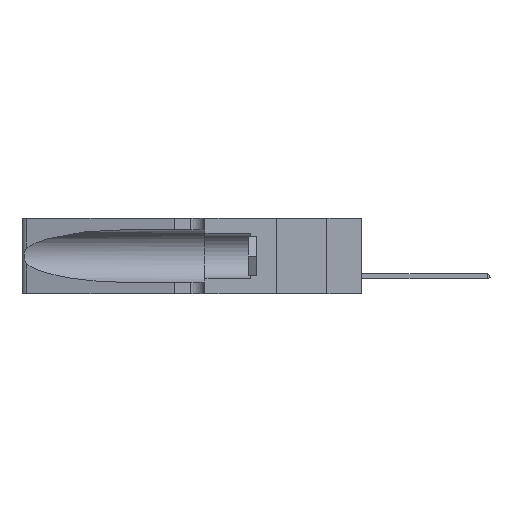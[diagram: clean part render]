
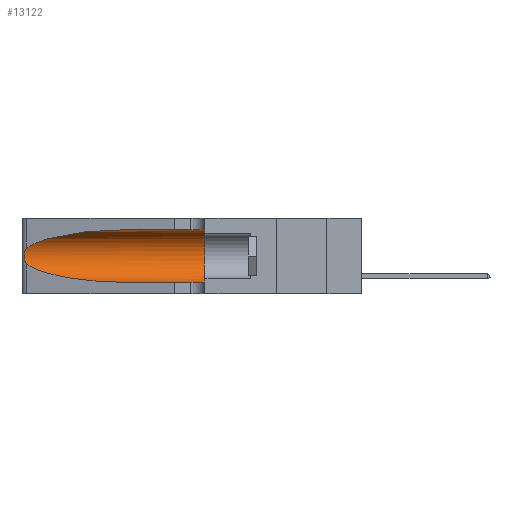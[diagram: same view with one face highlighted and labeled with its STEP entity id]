
A CAD part, left-side view. The second image highlights one B-rep face of the part: STEP entity #13122.
In plain terms, the highlighted cylindrical face has radius 3.308 mm (diameter 6.617 mm), a partial arc.
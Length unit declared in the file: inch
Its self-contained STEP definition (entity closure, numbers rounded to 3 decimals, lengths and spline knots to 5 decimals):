
#206 = DIRECTION ( 'NONE',  ( 0., 0., -1. ) ) ;
#385 = ORIENTED_EDGE ( 'NONE', *, *, #23380, .T. ) ;
#419 = CARTESIAN_POINT ( 'NONE',  ( 0.25854, 1.2359, 0.20912 ) ) ;
#603 = DIRECTION ( 'NONE',  ( 0., -1., 0. ) ) ;
#1376 = CARTESIAN_POINT ( 'NONE',  ( 0.1305, 0.35, 0.31525 ) ) ;
#1405 = VERTEX_POINT ( 'NONE', #1376 ) ;
#1760 = VECTOR ( 'NONE', #22590, 39.37008 ) ;
#1911 = CARTESIAN_POINT ( 'NONE',  ( 0.2373, 1.15595, 0.28018 ) ) ;
#2260 = EDGE_CURVE ( 'NONE', #12146, #18445, #20838, .T. ) ;
#2452 = CARTESIAN_POINT ( 'NONE',  ( 0.25639, 1.23186, 0.15144 ) ) ;
#2561 = CARTESIAN_POINT ( 'NONE',  ( 0.1305, 0.35, 0.05475 ) ) ;
#2890 = CARTESIAN_POINT ( 'NONE',  ( 0.25487, 1.22718, 0.14631 ) ) ;
#3723 = CARTESIAN_POINT ( 'NONE',  ( 0.1305, 1.61858, 0.185 ) ) ;
#3772 = CARTESIAN_POINT ( 'NONE',  ( 0.25487, 1.22718, 0.22369 ) ) ;
#4654 = CARTESIAN_POINT ( 'NONE',  ( 0.18966, 0.96281, 0.05475 ) ) ;
#5375 = LINE ( 'NONE', #6293, #9172 ) ;
#5584 = VERTEX_POINT ( 'NONE', #19292 ) ;
#5585 = DIRECTION ( 'NONE',  ( 0., -1., 0. ) ) ;
#6023 = CARTESIAN_POINT ( 'NONE',  ( 0.26018, 1.23835, 0.19895 ) ) ;
#6188 = CARTESIAN_POINT ( 'NONE',  ( 0.25555, 1.22993, 0.14849 ) ) ;
#6293 = CARTESIAN_POINT ( 'NONE',  ( 0.1305, 1.61858, 0.05475 ) ) ;
#6503 = CARTESIAN_POINT ( 'NONE',  ( 0.1305, 0.72297, 0.05475 ) ) ;
#6896 =( BOUNDED_CURVE ( )  B_SPLINE_CURVE ( 3, ( #16427, #7419, #1911, #3772 ),
 .UNSPECIFIED., .F., .T. ) 
 B_SPLINE_CURVE_WITH_KNOTS ( ( 4, 4 ),
 ( 1.5708, 2.84003 ),
 .UNSPECIFIED. ) 
 CURVE ( )  GEOMETRIC_REPRESENTATION_ITEM ( )  RATIONAL_B_SPLINE_CURVE ( ( 1., 0.87, 0.87, 1. ) ) 
 REPRESENTATION_ITEM ( '' )  );
#7058 = FACE_OUTER_BOUND ( 'NONE', #20716, .T. ) ;
#7419 = CARTESIAN_POINT ( 'NONE',  ( 0.18966, 0.96281, 0.31525 ) ) ;
#7560 = CARTESIAN_POINT ( 'NONE',  ( 0.1305, 0.72297, 0.31525 ) ) ;
#7807 = CIRCLE ( 'NONE', #8682, 0.13025 ) ;
#7890 = CARTESIAN_POINT ( 'NONE',  ( 0.26017, 1.23833, 0.17102 ) ) ;
#8385 = ORIENTED_EDGE ( 'NONE', *, *, #14040, .T. ) ;
#8682 = AXIS2_PLACEMENT_3D ( 'NONE', #15557, #16734, #20445 ) ;
#9172 = VECTOR ( 'NONE', #603, 39.37008 ) ;
#9507 = ORIENTED_EDGE ( 'NONE', *, *, #11261, .F. ) ;
#9690 = CARTESIAN_POINT ( 'NONE',  ( 0.25787, 1.23484, 0.2124 ) ) ;
#10184 = CARTESIAN_POINT ( 'NONE',  ( 0.25487, 1.22718, 0.14631 ) ) ;
#10285 = EDGE_CURVE ( 'NONE', #19319, #1405, #16267, .T. ) ;
#10358 = CARTESIAN_POINT ( 'NONE',  ( 0.25789, 1.23486, 0.15765 ) ) ;
#11046 = ORIENTED_EDGE ( 'NONE', *, *, #22620, .T. ) ;
#11257 = CARTESIAN_POINT ( 'NONE',  ( 0.25487, 1.22718, 0.14631 ) ) ;
#11261 = EDGE_CURVE ( 'NONE', #1405, #18204, #7807, .T. ) ;
#11281 = AXIS2_PLACEMENT_3D ( 'NONE', #3723, #5585, #206 ) ;
#12146 = VERTEX_POINT ( 'NONE', #15732 ) ;
#13122 = ADVANCED_FACE ( 'NONE', ( #7058 ), #19517, .F. ) ;
#13381 = CARTESIAN_POINT ( 'NONE',  ( 0.26075, 1.23896, 0.19203 ) ) ;
#13465 = CARTESIAN_POINT ( 'NONE',  ( 0.25856, 1.23593, 0.16098 ) ) ;
#13554 = CARTESIAN_POINT ( 'NONE',  ( 0.25487, 1.22718, 0.22369 ) ) ;
#13628 = CARTESIAN_POINT ( 'NONE',  ( 0.2373, 1.15595, 0.08982 ) ) ;
#14040 = EDGE_CURVE ( 'NONE', #19319, #12146, #6896, .T. ) ;
#15390 = ORIENTED_EDGE ( 'NONE', *, *, #2260, .T. ) ;
#15557 = CARTESIAN_POINT ( 'NONE',  ( 0.1305, 0.35, 0.185 ) ) ;
#15732 = CARTESIAN_POINT ( 'NONE',  ( 0.25487, 1.22718, 0.22369 ) ) ;
#16267 = LINE ( 'NONE', #22618, #1760 ) ;
#16427 = CARTESIAN_POINT ( 'NONE',  ( 0.1305, 0.72297, 0.31525 ) ) ;
#16734 = DIRECTION ( 'NONE',  ( 0., 1., 0. ) ) ;
#17267 = CARTESIAN_POINT ( 'NONE',  ( 0.25639, 1.23184, 0.21858 ) ) ;
#18204 = VERTEX_POINT ( 'NONE', #2561 ) ;
#18445 = VERTEX_POINT ( 'NONE', #11257 ) ;
#19292 = CARTESIAN_POINT ( 'NONE',  ( 0.1305, 0.72297, 0.05475 ) ) ;
#19319 = VERTEX_POINT ( 'NONE', #7560 ) ;
#19505 =( BOUNDED_CURVE ( )  B_SPLINE_CURVE ( 3, ( #10184, #13628, #4654, #6503 ),
 .UNSPECIFIED., .F., .T. ) 
 B_SPLINE_CURVE_WITH_KNOTS ( ( 4, 4 ),
 ( 3.44316, 4.71239 ),
 .UNSPECIFIED. ) 
 CURVE ( )  GEOMETRIC_REPRESENTATION_ITEM ( )  RATIONAL_B_SPLINE_CURVE ( ( 1., 0.87, 0.87, 1. ) ) 
 REPRESENTATION_ITEM ( '' )  );
#19517 = CYLINDRICAL_SURFACE ( 'NONE', #11281, 0.13025 ) ;
#20445 = DIRECTION ( 'NONE',  ( 0., 0., 1. ) ) ;
#20716 = EDGE_LOOP ( 'NONE', ( #8385, #15390, #11046, #385, #9507, #23960 ) ) ;
#20838 = B_SPLINE_CURVE_WITH_KNOTS ( 'NONE', 3,
 ( #13554, #21402, #17267, #9690, #419, #6023, #13381, #23295, #7890, #13465, #10358, #2452, #6188, #2890 ),
 .UNSPECIFIED., .F., .F.,
 ( 4, 2, 2, 2, 2, 2, 4 ),
 ( 0., 0.00027, 0.00053, 0.00107, 0.0016, 0.00187, 0.00214 ),
 .UNSPECIFIED. ) ;
#21402 = CARTESIAN_POINT ( 'NONE',  ( 0.25555, 1.22994, 0.2215 ) ) ;
#22590 = DIRECTION ( 'NONE',  ( 0., -1., 0. ) ) ;
#22618 = CARTESIAN_POINT ( 'NONE',  ( 0.1305, 1.61858, 0.31525 ) ) ;
#22620 = EDGE_CURVE ( 'NONE', #18445, #5584, #19505, .T. ) ;
#23295 = CARTESIAN_POINT ( 'NONE',  ( 0.26075, 1.23896, 0.178 ) ) ;
#23380 = EDGE_CURVE ( 'NONE', #5584, #18204, #5375, .T. ) ;
#23960 = ORIENTED_EDGE ( 'NONE', *, *, #10285, .F. ) ;
